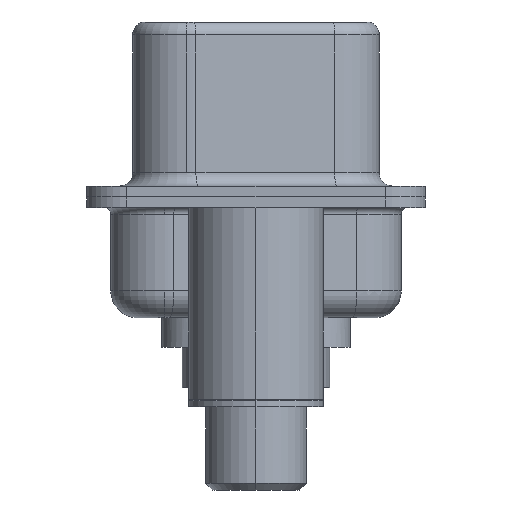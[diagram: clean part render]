
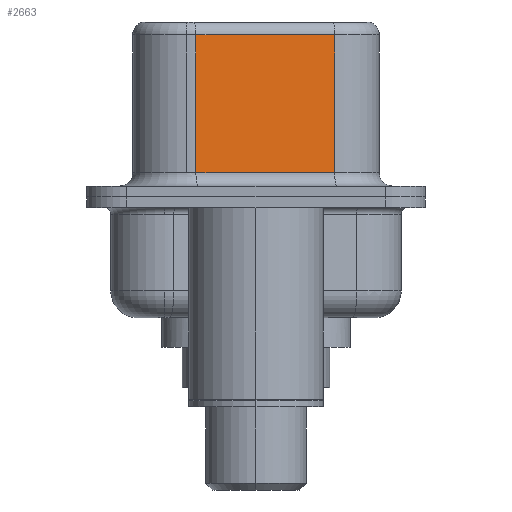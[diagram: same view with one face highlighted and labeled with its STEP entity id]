
A CAD part, left-side view. The second image highlights one B-rep face of the part: STEP entity #2663.
In plain terms, the highlighted planar face has unit normal (-0.985, -0.174, 0).
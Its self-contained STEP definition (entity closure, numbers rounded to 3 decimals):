
#518 = LINE ( 'NONE', #12920, #10158 ) ;
#1640 = ORIENTED_EDGE ( 'NONE', *, *, #3453, .T. ) ;
#2204 = LINE ( 'NONE', #11947, #14997 ) ;
#2466 = ORIENTED_EDGE ( 'NONE', *, *, #16115, .T. ) ;
#2598 = VECTOR ( 'NONE', #7924, 1000. ) ;
#2663 = ADVANCED_FACE ( 'NONE', ( #13138 ), #6389, .F. ) ;
#3453 = EDGE_CURVE ( 'NONE', #12631, #7498, #12921, .T. ) ;
#3698 = VECTOR ( 'NONE', #7456, 1000. ) ;
#4095 = LINE ( 'NONE', #12400, #3698 ) ;
#5286 = EDGE_LOOP ( 'NONE', ( #5571, #2466, #1640, #14112 ) ) ;
#5571 = ORIENTED_EDGE ( 'NONE', *, *, #7183, .F. ) ;
#6376 = EDGE_CURVE ( 'NONE', #7498, #13930, #518, .T. ) ;
#6389 = PLANE ( 'NONE',  #8587 ) ;
#6972 = CARTESIAN_POINT ( 'NONE',  ( 3.655, 2.233, 6.52 ) ) ;
#7183 = EDGE_CURVE ( 'NONE', #10717, #13930, #4095, .T. ) ;
#7456 = DIRECTION ( 'NONE',  ( 0., 0., -1. ) ) ;
#7498 = VERTEX_POINT ( 'NONE', #13065 ) ;
#7924 = DIRECTION ( 'NONE',  ( 0., 0., -1. ) ) ;
#8587 = AXIS2_PLACEMENT_3D ( 'NONE', #10113, #10712, #13832 ) ;
#10113 = CARTESIAN_POINT ( 'NONE',  ( 4.565, -2.927, 6.52 ) ) ;
#10158 = VECTOR ( 'NONE', #12332, 1000. ) ;
#10712 = DIRECTION ( 'NONE',  ( 0.985, 0.174, 0. ) ) ;
#10717 = VERTEX_POINT ( 'NONE', #13096 ) ;
#11947 = CARTESIAN_POINT ( 'NONE',  ( 4.565, -2.927, 6.02 ) ) ;
#11998 = DIRECTION ( 'NONE',  ( -0.174, 0.985, 0. ) ) ;
#12332 = DIRECTION ( 'NONE',  ( 0.174, -0.985, 0. ) ) ;
#12400 = CARTESIAN_POINT ( 'NONE',  ( 4.565, -2.927, 6.52 ) ) ;
#12631 = VERTEX_POINT ( 'NONE', #14472 ) ;
#12920 = CARTESIAN_POINT ( 'NONE',  ( 4.565, -2.927, 0.9 ) ) ;
#12921 = LINE ( 'NONE', #6972, #2598 ) ;
#13065 = CARTESIAN_POINT ( 'NONE',  ( 3.655, 2.233, 0.9 ) ) ;
#13096 = CARTESIAN_POINT ( 'NONE',  ( 4.565, -2.927, 6.02 ) ) ;
#13138 = FACE_OUTER_BOUND ( 'NONE', #5286, .T. ) ;
#13558 = CARTESIAN_POINT ( 'NONE',  ( 4.565, -2.927, 0.9 ) ) ;
#13832 = DIRECTION ( 'NONE',  ( -0.174, 0.985, 0. ) ) ;
#13930 = VERTEX_POINT ( 'NONE', #13558 ) ;
#14112 = ORIENTED_EDGE ( 'NONE', *, *, #6376, .T. ) ;
#14472 = CARTESIAN_POINT ( 'NONE',  ( 3.655, 2.233, 6.02 ) ) ;
#14997 = VECTOR ( 'NONE', #11998, 1000. ) ;
#16115 = EDGE_CURVE ( 'NONE', #10717, #12631, #2204, .T. ) ;
